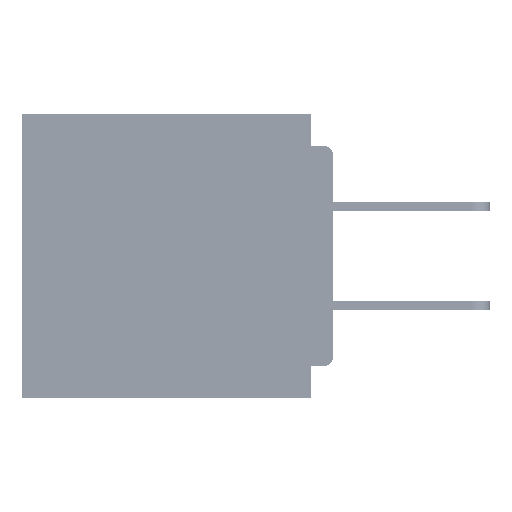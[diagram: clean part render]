
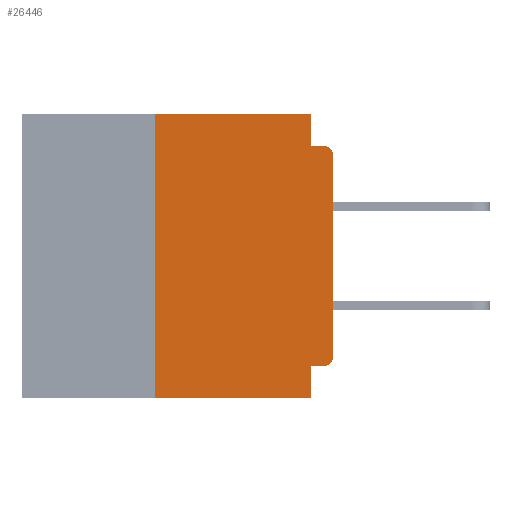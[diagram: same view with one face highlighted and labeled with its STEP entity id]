
A CAD part, left-side view. The second image highlights one B-rep face of the part: STEP entity #26446.
In plain terms, the highlighted planar face has unit normal (-1, 0, 0).
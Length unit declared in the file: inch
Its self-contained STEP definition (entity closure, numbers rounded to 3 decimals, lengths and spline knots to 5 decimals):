
#240 = LINE ( 'NONE', #13812, #24180 ) ;
#2530 = LINE ( 'NONE', #24055, #69876 ) ;
#3301 = EDGE_CURVE ( 'NONE', #27311, #12690, #4088, .T. ) ;
#4088 = LINE ( 'NONE', #38555, #16926 ) ;
#4177 = CARTESIAN_POINT ( 'NONE',  ( 0., 0.437, -0.4 ) ) ;
#4918 = FACE_OUTER_BOUND ( 'NONE', #23815, .T. ) ;
#4963 = DIRECTION ( 'NONE',  ( 0., 0., -1. ) ) ;
#5735 = ORIENTED_EDGE ( 'NONE', *, *, #40001, .F. ) ;
#7801 = DIRECTION ( 'NONE',  ( 0., -1., 0. ) ) ;
#8304 = VECTOR ( 'NONE', #65802, 39.37008 ) ;
#8557 = ORIENTED_EDGE ( 'NONE', *, *, #3301, .F. ) ;
#11211 = CARTESIAN_POINT ( 'NONE',  ( 0., 0.437, 0. ) ) ;
#11257 = VERTEX_POINT ( 'NONE', #50016 ) ;
#11471 = VECTOR ( 'NONE', #60444, 39.37008 ) ;
#12690 = VERTEX_POINT ( 'NONE', #68374 ) ;
#13341 = DIRECTION ( 'NONE',  ( -1., 0., 0. ) ) ;
#13812 = CARTESIAN_POINT ( 'NONE',  ( 0., 0.25, -0.4 ) ) ;
#15257 = ORIENTED_EDGE ( 'NONE', *, *, #30972, .F. ) ;
#15280 = EDGE_CURVE ( 'NONE', #27311, #11257, #47288, .T. ) ;
#15406 = EDGE_CURVE ( 'NONE', #11257, #50179, #65927, .T. ) ;
#16777 = EDGE_CURVE ( 'NONE', #50179, #49866, #20645, .T. ) ;
#16859 = DIRECTION ( 'NONE',  ( 0., 1., 0. ) ) ;
#16926 = VECTOR ( 'NONE', #16859, 39.37008 ) ;
#16963 = EDGE_CURVE ( 'NONE', #48959, #41686, #53803, .T. ) ;
#20154 = LINE ( 'NONE', #23404, #21870 ) ;
#20645 = CIRCLE ( 'NONE', #68391, 0.015 ) ;
#21466 = VECTOR ( 'NONE', #36888, 39.37008 ) ;
#21680 = CARTESIAN_POINT ( 'NONE',  ( 0., 0.437, 0. ) ) ;
#21870 = VECTOR ( 'NONE', #61451, 39.37008 ) ;
#21931 = ORIENTED_EDGE ( 'NONE', *, *, #62289, .F. ) ;
#22412 = CARTESIAN_POINT ( 'NONE',  ( 0., 0., 0. ) ) ;
#22910 = VERTEX_POINT ( 'NONE', #40403 ) ;
#23404 = CARTESIAN_POINT ( 'NONE',  ( 0., 0.031, 0. ) ) ;
#23815 = EDGE_LOOP ( 'NONE', ( #46609, #26083, #5735, #64947, #15257, #21931, #52731, #45421, #8557, #60911 ) ) ;
#24055 = CARTESIAN_POINT ( 'NONE',  ( 0., 0., -0.045 ) ) ;
#24180 = VECTOR ( 'NONE', #46446, 39.37008 ) ;
#26083 = ORIENTED_EDGE ( 'NONE', *, *, #16777, .T. ) ;
#26446 = ADVANCED_FACE ( 'NONE', ( #4918 ), #59717, .F. ) ;
#27161 = DIRECTION ( 'NONE',  ( 1., 0., 0. ) ) ;
#27311 = VERTEX_POINT ( 'NONE', #39411 ) ;
#28978 = CARTESIAN_POINT ( 'NONE',  ( 0., 0.015, -0.045 ) ) ;
#30731 = VECTOR ( 'NONE', #44066, 39.37008 ) ;
#30972 = EDGE_CURVE ( 'NONE', #33675, #63035, #59626, .T. ) ;
#33236 = CARTESIAN_POINT ( 'NONE',  ( 0., 0.031, -0.4 ) ) ;
#33675 = VERTEX_POINT ( 'NONE', #47540 ) ;
#36888 = DIRECTION ( 'NONE',  ( 0., -1., 0. ) ) ;
#37307 = LINE ( 'NONE', #33236, #8304 ) ;
#37658 = DIRECTION ( 'NONE',  ( -1., 0., 0. ) ) ;
#38555 = CARTESIAN_POINT ( 'NONE',  ( 0., 0., -0.355 ) ) ;
#39411 = CARTESIAN_POINT ( 'NONE',  ( 0., 0.015, -0.355 ) ) ;
#40001 = EDGE_CURVE ( 'NONE', #22910, #49866, #2530, .T. ) ;
#40403 = CARTESIAN_POINT ( 'NONE',  ( 0., 0.031, -0.045 ) ) ;
#41686 = VERTEX_POINT ( 'NONE', #65392 ) ;
#42717 = CARTESIAN_POINT ( 'NONE',  ( 0., 0., -0.06 ) ) ;
#44066 = DIRECTION ( 'NONE',  ( 0., -1., 0. ) ) ;
#44659 = AXIS2_PLACEMENT_3D ( 'NONE', #70228, #37658, #4963 ) ;
#45421 = ORIENTED_EDGE ( 'NONE', *, *, #59578, .F. ) ;
#45953 = CARTESIAN_POINT ( 'NONE',  ( 0., 0.015, -0.06 ) ) ;
#46446 = DIRECTION ( 'NONE',  ( 0., 0., 1. ) ) ;
#46609 = ORIENTED_EDGE ( 'NONE', *, *, #15406, .T. ) ;
#46840 = CARTESIAN_POINT ( 'NONE',  ( 0., 0.031, 0. ) ) ;
#47288 = CIRCLE ( 'NONE', #44659, 0.015 ) ;
#47540 = CARTESIAN_POINT ( 'NONE',  ( 0., 0.25, 0. ) ) ;
#48959 = VERTEX_POINT ( 'NONE', #63298 ) ;
#49866 = VERTEX_POINT ( 'NONE', #28978 ) ;
#50016 = CARTESIAN_POINT ( 'NONE',  ( 0., 0., -0.34 ) ) ;
#50179 = VERTEX_POINT ( 'NONE', #42717 ) ;
#51420 = DIRECTION ( 'NONE',  ( 0., 0., -1. ) ) ;
#52731 = ORIENTED_EDGE ( 'NONE', *, *, #16963, .T. ) ;
#53803 = LINE ( 'NONE', #4177, #21466 ) ;
#59578 = EDGE_CURVE ( 'NONE', #12690, #41686, #37307, .T. ) ;
#59626 = LINE ( 'NONE', #11211, #30731 ) ;
#59717 = PLANE ( 'NONE',  #62252 ) ;
#60341 = EDGE_CURVE ( 'NONE', #63035, #22910, #20154, .T. ) ;
#60444 = DIRECTION ( 'NONE',  ( 0., 0., 1. ) ) ;
#60911 = ORIENTED_EDGE ( 'NONE', *, *, #15280, .T. ) ;
#61451 = DIRECTION ( 'NONE',  ( 0., 0., -1. ) ) ;
#62252 = AXIS2_PLACEMENT_3D ( 'NONE', #21680, #27161, #65172 ) ;
#62289 = EDGE_CURVE ( 'NONE', #48959, #33675, #240, .T. ) ;
#63035 = VERTEX_POINT ( 'NONE', #46840 ) ;
#63298 = CARTESIAN_POINT ( 'NONE',  ( 0., 0.25, -0.4 ) ) ;
#64947 = ORIENTED_EDGE ( 'NONE', *, *, #60341, .F. ) ;
#65172 = DIRECTION ( 'NONE',  ( 0., 0., -1. ) ) ;
#65392 = CARTESIAN_POINT ( 'NONE',  ( 0., 0.031, -0.4 ) ) ;
#65802 = DIRECTION ( 'NONE',  ( 0., 0., -1. ) ) ;
#65927 = LINE ( 'NONE', #22412, #11471 ) ;
#68374 = CARTESIAN_POINT ( 'NONE',  ( 0., 0.031, -0.355 ) ) ;
#68391 = AXIS2_PLACEMENT_3D ( 'NONE', #45953, #13341, #51420 ) ;
#69876 = VECTOR ( 'NONE', #7801, 39.37008 ) ;
#70228 = CARTESIAN_POINT ( 'NONE',  ( 0., 0.015, -0.34 ) ) ;
